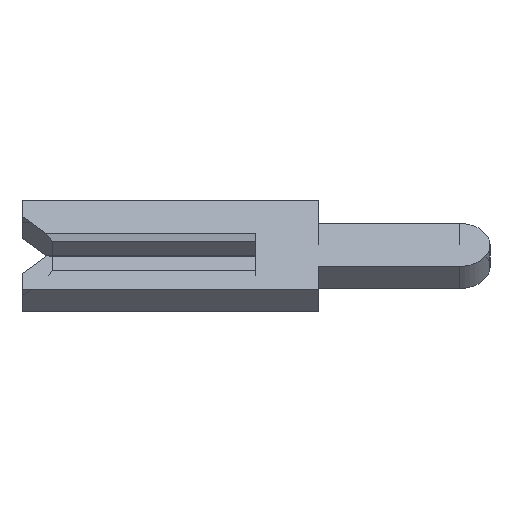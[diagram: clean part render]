
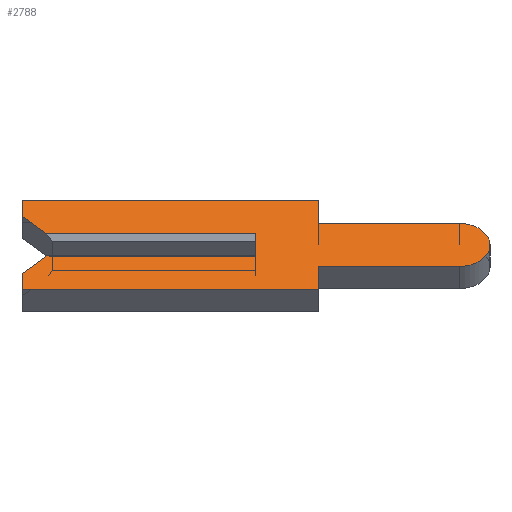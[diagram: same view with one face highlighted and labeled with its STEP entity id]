
A CAD part, left-side view. The second image highlights one B-rep face of the part: STEP entity #2788.
In plain terms, the highlighted face is planar.
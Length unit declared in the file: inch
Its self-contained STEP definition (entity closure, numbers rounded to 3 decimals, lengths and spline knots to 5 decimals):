
#36 = LINE ( 'NONE', #1496, #752 ) ;
#37 = VECTOR ( 'NONE', #2322, 39.37008 ) ;
#59 = EDGE_CURVE ( 'NONE', #1159, #2402, #2496, .T. ) ;
#73 = VECTOR ( 'NONE', #2568, 39.37008 ) ;
#74 = VERTEX_POINT ( 'NONE', #626 ) ;
#88 = LINE ( 'NONE', #1203, #1928 ) ;
#97 = VERTEX_POINT ( 'NONE', #400 ) ;
#177 = VECTOR ( 'NONE', #1974, 39.37008 ) ;
#180 = ORIENTED_EDGE ( 'NONE', *, *, #2624, .F. ) ;
#243 = CARTESIAN_POINT ( 'NONE',  ( -0.01, 0.15, -0.026 ) ) ;
#282 = EDGE_CURVE ( 'NONE', #1326, #2402, #2267, .T. ) ;
#310 = ORIENTED_EDGE ( 'NONE', *, *, #2846, .F. ) ;
#313 = DIRECTION ( 'NONE',  ( 0., 0., -1. ) ) ;
#322 = LINE ( 'NONE', #1805, #2298 ) ;
#325 = LINE ( 'NONE', #970, #1427 ) ;
#327 = VERTEX_POINT ( 'NONE', #930 ) ;
#360 = VECTOR ( 'NONE', #1111, 39.37008 ) ;
#395 = ORIENTED_EDGE ( 'NONE', *, *, #1743, .F. ) ;
#400 = CARTESIAN_POINT ( 'NONE',  ( -0.01, -0.04, 0.04 ) ) ;
#434 = DIRECTION ( 'NONE',  ( 0., 1., 0. ) ) ;
#474 = EDGE_CURVE ( 'NONE', #2706, #721, #2898, .T. ) ;
#492 = CARTESIAN_POINT ( 'NONE',  ( -0.01, 0.134, -0.01 ) ) ;
#513 = DIRECTION ( 'NONE',  ( 0., 1., 0. ) ) ;
#522 = CARTESIAN_POINT ( 'NONE',  ( -0.01, -0.1305, -0.0195 ) ) ;
#538 = LINE ( 'NONE', #565, #177 ) ;
#548 = ORIENTED_EDGE ( 'NONE', *, *, #577, .F. ) ;
#565 = CARTESIAN_POINT ( 'NONE',  ( -0.01, 0.1305, -0.0065 ) ) ;
#573 = ORIENTED_EDGE ( 'NONE', *, *, #2139, .F. ) ;
#577 = EDGE_CURVE ( 'NONE', #1198, #1326, #1570, .T. ) ;
#626 = CARTESIAN_POINT ( 'NONE',  ( -0.01, 0.15, 0.04 ) ) ;
#642 = ORIENTED_EDGE ( 'NONE', *, *, #1489, .F. ) ;
#721 = VERTEX_POINT ( 'NONE', #243 ) ;
#752 = VECTOR ( 'NONE', #2674, 39.37008 ) ;
#825 = VECTOR ( 'NONE', #923, 39.37008 ) ;
#904 = ORIENTED_EDGE ( 'NONE', *, *, #2941, .F. ) ;
#907 = ORIENTED_EDGE ( 'NONE', *, *, #474, .F. ) ;
#923 = DIRECTION ( 'NONE',  ( 0., 0., 1. ) ) ;
#930 = CARTESIAN_POINT ( 'NONE',  ( -0.01, -0.04, -0.04 ) ) ;
#936 = FACE_OUTER_BOUND ( 'NONE', #2603, .T. ) ;
#941 = VERTEX_POINT ( 'NONE', #522 ) ;
#943 = EDGE_CURVE ( 'NONE', #2286, #941, #2007, .T. ) ;
#954 = CARTESIAN_POINT ( 'NONE',  ( -0.01, -0.1305, 0. ) ) ;
#970 = CARTESIAN_POINT ( 'NONE',  ( -0.01, 0.15, 0.026 ) ) ;
#973 = LINE ( 'NONE', #1357, #2004 ) ;
#974 = ORIENTED_EDGE ( 'NONE', *, *, #1428, .F. ) ;
#1059 = EDGE_CURVE ( 'NONE', #2926, #74, #325, .T. ) ;
#1105 = DIRECTION ( 'NONE',  ( 0., -1., 0. ) ) ;
#1111 = DIRECTION ( 'NONE',  ( 0., -1., 0. ) ) ;
#1127 = LINE ( 'NONE', #1561, #2086 ) ;
#1159 = VERTEX_POINT ( 'NONE', #1186 ) ;
#1171 = VERTEX_POINT ( 'NONE', #1456 ) ;
#1186 = CARTESIAN_POINT ( 'NONE',  ( -0.01, 0.134, 0.01 ) ) ;
#1188 = EDGE_CURVE ( 'NONE', #74, #97, #1320, .T. ) ;
#1198 = VERTEX_POINT ( 'NONE', #492 ) ;
#1203 = CARTESIAN_POINT ( 'NONE',  ( -0.01, -0.04, -0.0195 ) ) ;
#1226 = DIRECTION ( 'NONE',  ( 1., 0., 0. ) ) ;
#1283 = CARTESIAN_POINT ( 'NONE',  ( -0.01, -0.04, -0.04 ) ) ;
#1294 = ORIENTED_EDGE ( 'NONE', *, *, #1059, .F. ) ;
#1320 = LINE ( 'NONE', #2830, #2418 ) ;
#1321 = CARTESIAN_POINT ( 'NONE',  ( -0.01, -0.04, 0.0195 ) ) ;
#1326 = VERTEX_POINT ( 'NONE', #2119 ) ;
#1357 = CARTESIAN_POINT ( 'NONE',  ( -0.01, 0.15, -0.04 ) ) ;
#1423 = DIRECTION ( 'NONE',  ( 0., -1., 0. ) ) ;
#1427 = VECTOR ( 'NONE', #2600, 39.37008 ) ;
#1428 = EDGE_CURVE ( 'NONE', #941, #1171, #88, .T. ) ;
#1456 = CARTESIAN_POINT ( 'NONE',  ( -0.01, -0.04, -0.0195 ) ) ;
#1489 = EDGE_CURVE ( 'NONE', #721, #1198, #538, .T. ) ;
#1496 = CARTESIAN_POINT ( 'NONE',  ( -0.01, -0.04, 0.04 ) ) ;
#1540 = CARTESIAN_POINT ( 'NONE',  ( -0.01, 0.15, 0.026 ) ) ;
#1545 = AXIS2_PLACEMENT_3D ( 'NONE', #2501, #2289, #2527 ) ;
#1553 = CARTESIAN_POINT ( 'NONE',  ( -0.01, -0.1305, 0.0195 ) ) ;
#1561 = CARTESIAN_POINT ( 'NONE',  ( -0.01, 0.1305, 0.0065 ) ) ;
#1570 = LINE ( 'NONE', #2579, #73 ) ;
#1602 = PLANE ( 'NONE',  #1545 ) ;
#1722 = AXIS2_PLACEMENT_3D ( 'NONE', #954, #1226, #1922 ) ;
#1743 = EDGE_CURVE ( 'NONE', #97, #2255, #36, .T. ) ;
#1778 = CARTESIAN_POINT ( 'NONE',  ( -0.01, 0., 0.01 ) ) ;
#1805 = CARTESIAN_POINT ( 'NONE',  ( -0.01, -0.04, 0.0195 ) ) ;
#1922 = DIRECTION ( 'NONE',  ( 0., 0., -1. ) ) ;
#1928 = VECTOR ( 'NONE', #513, 39.37008 ) ;
#1974 = DIRECTION ( 'NONE',  ( 0., -0.707, 0.707 ) ) ;
#2004 = VECTOR ( 'NONE', #434, 39.37008 ) ;
#2007 = CIRCLE ( 'NONE', #1722, 0.0195 ) ;
#2041 = ORIENTED_EDGE ( 'NONE', *, *, #59, .T. ) ;
#2086 = VECTOR ( 'NONE', #2697, 39.37008 ) ;
#2091 = CARTESIAN_POINT ( 'NONE',  ( -0.01, 0., 0.0065 ) ) ;
#2104 = CARTESIAN_POINT ( 'NONE',  ( -0.01, 0.15, -0.026 ) ) ;
#2119 = CARTESIAN_POINT ( 'NONE',  ( -0.01, 0., -0.01 ) ) ;
#2139 = EDGE_CURVE ( 'NONE', #1171, #327, #2744, .T. ) ;
#2241 = ORIENTED_EDGE ( 'NONE', *, *, #1188, .F. ) ;
#2255 = VERTEX_POINT ( 'NONE', #1321 ) ;
#2267 = LINE ( 'NONE', #2091, #37 ) ;
#2286 = VERTEX_POINT ( 'NONE', #1553 ) ;
#2289 = DIRECTION ( 'NONE',  ( 1., 0., 0. ) ) ;
#2298 = VECTOR ( 'NONE', #1105, 39.37008 ) ;
#2322 = DIRECTION ( 'NONE',  ( 0., 0., 1. ) ) ;
#2349 = ORIENTED_EDGE ( 'NONE', *, *, #282, .F. ) ;
#2402 = VERTEX_POINT ( 'NONE', #1778 ) ;
#2418 = VECTOR ( 'NONE', #1423, 39.37008 ) ;
#2496 = LINE ( 'NONE', #2746, #360 ) ;
#2501 = CARTESIAN_POINT ( 'NONE',  ( -0.01, -0.1305, 0. ) ) ;
#2527 = DIRECTION ( 'NONE',  ( 0., 0., -1. ) ) ;
#2568 = DIRECTION ( 'NONE',  ( 0., -1., 0. ) ) ;
#2579 = CARTESIAN_POINT ( 'NONE',  ( -0.01, -0.1305, -0.01 ) ) ;
#2600 = DIRECTION ( 'NONE',  ( 0., 0., 1. ) ) ;
#2603 = EDGE_LOOP ( 'NONE', ( #2041, #2349, #548, #642, #907, #310, #573, #974, #2666, #904, #395, #2241, #1294, #180 ) ) ;
#2624 = EDGE_CURVE ( 'NONE', #1159, #2926, #1127, .T. ) ;
#2666 = ORIENTED_EDGE ( 'NONE', *, *, #943, .F. ) ;
#2674 = DIRECTION ( 'NONE',  ( 0., 0., -1. ) ) ;
#2697 = DIRECTION ( 'NONE',  ( 0., 0.707, 0.707 ) ) ;
#2706 = VERTEX_POINT ( 'NONE', #2950 ) ;
#2710 = VECTOR ( 'NONE', #313, 39.37008 ) ;
#2744 = LINE ( 'NONE', #1283, #2710 ) ;
#2746 = CARTESIAN_POINT ( 'NONE',  ( -0.01, 0.15, 0.01 ) ) ;
#2788 = ADVANCED_FACE ( 'NONE', ( #936 ), #1602, .F. ) ;
#2830 = CARTESIAN_POINT ( 'NONE',  ( -0.01, 0.15, 0.04 ) ) ;
#2846 = EDGE_CURVE ( 'NONE', #327, #2706, #973, .T. ) ;
#2898 = LINE ( 'NONE', #2104, #825 ) ;
#2926 = VERTEX_POINT ( 'NONE', #1540 ) ;
#2941 = EDGE_CURVE ( 'NONE', #2255, #2286, #322, .T. ) ;
#2950 = CARTESIAN_POINT ( 'NONE',  ( -0.01, 0.15, -0.04 ) ) ;
